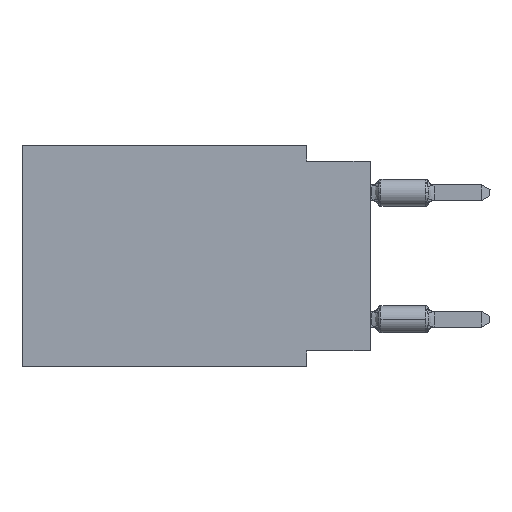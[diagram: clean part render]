
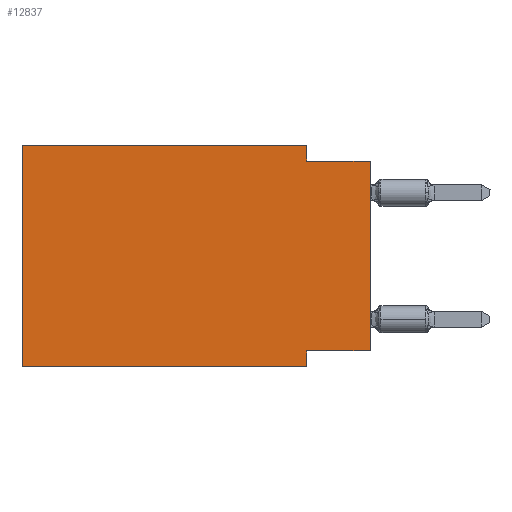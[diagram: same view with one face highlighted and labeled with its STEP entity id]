
A CAD part, left-side view. The second image highlights one B-rep face of the part: STEP entity #12837.
In plain terms, the highlighted planar face has unit normal (-1, 0, 0).
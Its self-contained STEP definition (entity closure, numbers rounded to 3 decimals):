
#1103 = PLANE ( 'NONE',  #6966 ) ;
#1621 = CARTESIAN_POINT ( 'NONE',  ( 0., 0., -0.635 ) ) ;
#2023 = ORIENTED_EDGE ( 'NONE', *, *, #9951, .T. ) ;
#2325 = LINE ( 'NONE', #35380, #24742 ) ;
#2414 = LINE ( 'NONE', #32204, #32189 ) ;
#2681 = DIRECTION ( 'NONE',  ( 0., 0., 1. ) ) ;
#2728 = LINE ( 'NONE', #8503, #26815 ) ;
#3178 = VERTEX_POINT ( 'NONE', #7827 ) ;
#3295 = DIRECTION ( 'NONE',  ( 0., -1., 0. ) ) ;
#3727 = CARTESIAN_POINT ( 'NONE',  ( 0., 2.54, 0. ) ) ;
#3992 = DIRECTION ( 'NONE',  ( 0., 0., -1. ) ) ;
#4906 = CARTESIAN_POINT ( 'NONE',  ( 0., 2.54, -8.89 ) ) ;
#5496 = DIRECTION ( 'NONE',  ( 0., 0., -1. ) ) ;
#5812 = CARTESIAN_POINT ( 'NONE',  ( 0., 13.97, -8.89 ) ) ;
#6497 = EDGE_CURVE ( 'NONE', #13696, #20800, #2728, .T. ) ;
#6539 = FACE_OUTER_BOUND ( 'NONE', #21527, .T. ) ;
#6740 = LINE ( 'NONE', #17583, #24467 ) ;
#6859 = LINE ( 'NONE', #12635, #31908 ) ;
#6966 = AXIS2_PLACEMENT_3D ( 'NONE', #14470, #23130, #3992 ) ;
#7316 = ORIENTED_EDGE ( 'NONE', *, *, #10453, .T. ) ;
#7827 = CARTESIAN_POINT ( 'NONE',  ( 0., 2.54, -8.255 ) ) ;
#8329 = VECTOR ( 'NONE', #32636, 1000. ) ;
#8503 = CARTESIAN_POINT ( 'NONE',  ( 0., 2.54, 0. ) ) ;
#8764 = ORIENTED_EDGE ( 'NONE', *, *, #19753, .F. ) ;
#9951 = EDGE_CURVE ( 'NONE', #21202, #30269, #6740, .T. ) ;
#10282 = VERTEX_POINT ( 'NONE', #20053 ) ;
#10453 = EDGE_CURVE ( 'NONE', #28560, #13000, #21439, .T. ) ;
#10890 = LINE ( 'NONE', #21736, #21448 ) ;
#12635 = CARTESIAN_POINT ( 'NONE',  ( 0., 13.97, 0. ) ) ;
#12837 = ADVANCED_FACE ( 'NONE', ( #6539 ), #1103, .F. ) ;
#12958 = DIRECTION ( 'NONE',  ( 0., -1., 0. ) ) ;
#13000 = VERTEX_POINT ( 'NONE', #1621 ) ;
#13696 = VERTEX_POINT ( 'NONE', #3727 ) ;
#13879 = ORIENTED_EDGE ( 'NONE', *, *, #16661, .F. ) ;
#14470 = CARTESIAN_POINT ( 'NONE',  ( 0., 13.97, 0. ) ) ;
#14740 = ORIENTED_EDGE ( 'NONE', *, *, #23909, .F. ) ;
#15850 = CARTESIAN_POINT ( 'NONE',  ( 0., 0., 0. ) ) ;
#16661 = EDGE_CURVE ( 'NONE', #28560, #3178, #2414, .T. ) ;
#17583 = CARTESIAN_POINT ( 'NONE',  ( 0., 13.97, -8.89 ) ) ;
#17679 = EDGE_CURVE ( 'NONE', #21202, #10282, #2325, .T. ) ;
#18196 = LINE ( 'NONE', #23789, #34085 ) ;
#18271 = ORIENTED_EDGE ( 'NONE', *, *, #21338, .F. ) ;
#19753 = EDGE_CURVE ( 'NONE', #10282, #13696, #6859, .T. ) ;
#20053 = CARTESIAN_POINT ( 'NONE',  ( 0., 13.97, 0. ) ) ;
#20800 = VERTEX_POINT ( 'NONE', #25155 ) ;
#21202 = VERTEX_POINT ( 'NONE', #5812 ) ;
#21338 = EDGE_CURVE ( 'NONE', #20800, #13000, #18196, .T. ) ;
#21439 = LINE ( 'NONE', #15850, #8329 ) ;
#21448 = VECTOR ( 'NONE', #5496, 1000. ) ;
#21527 = EDGE_LOOP ( 'NONE', ( #7316, #18271, #33209, #8764, #31174, #2023, #14740, #13879 ) ) ;
#21736 = CARTESIAN_POINT ( 'NONE',  ( 0., 2.54, -8.89 ) ) ;
#23130 = DIRECTION ( 'NONE',  ( 1., 0., 0. ) ) ;
#23642 = DIRECTION ( 'NONE',  ( 0., -1., 0. ) ) ;
#23789 = CARTESIAN_POINT ( 'NONE',  ( 0., 0., -0.635 ) ) ;
#23909 = EDGE_CURVE ( 'NONE', #3178, #30269, #10890, .T. ) ;
#24439 = DIRECTION ( 'NONE',  ( 0., 1., 0. ) ) ;
#24467 = VECTOR ( 'NONE', #3295, 1000. ) ;
#24742 = VECTOR ( 'NONE', #2681, 1000. ) ;
#25016 = CARTESIAN_POINT ( 'NONE',  ( 0., 0., -8.255 ) ) ;
#25155 = CARTESIAN_POINT ( 'NONE',  ( 0., 2.54, -0.635 ) ) ;
#26815 = VECTOR ( 'NONE', #33081, 1000. ) ;
#28560 = VERTEX_POINT ( 'NONE', #25016 ) ;
#30269 = VERTEX_POINT ( 'NONE', #4906 ) ;
#31174 = ORIENTED_EDGE ( 'NONE', *, *, #17679, .F. ) ;
#31908 = VECTOR ( 'NONE', #23642, 1000. ) ;
#32189 = VECTOR ( 'NONE', #24439, 1000. ) ;
#32204 = CARTESIAN_POINT ( 'NONE',  ( 0., 0., -8.255 ) ) ;
#32636 = DIRECTION ( 'NONE',  ( 0., 0., 1. ) ) ;
#33081 = DIRECTION ( 'NONE',  ( 0., 0., -1. ) ) ;
#33209 = ORIENTED_EDGE ( 'NONE', *, *, #6497, .F. ) ;
#34085 = VECTOR ( 'NONE', #12958, 1000. ) ;
#35380 = CARTESIAN_POINT ( 'NONE',  ( 0., 13.97, 0. ) ) ;
